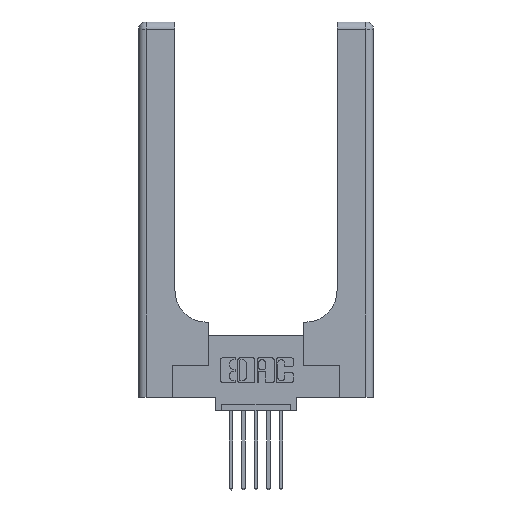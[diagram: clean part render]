
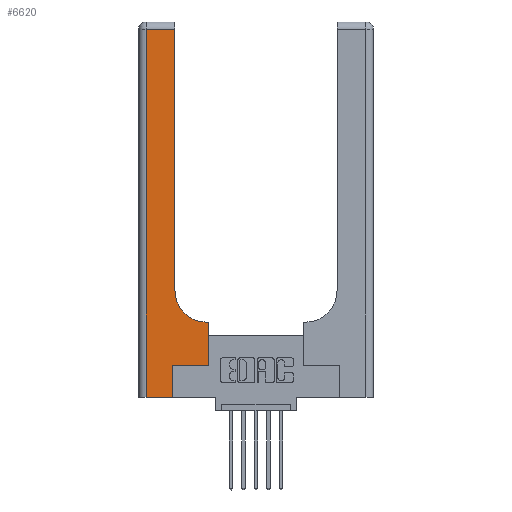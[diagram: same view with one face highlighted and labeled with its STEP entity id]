
A CAD part, top view. The second image highlights one B-rep face of the part: STEP entity #6620.
In plain terms, the highlighted planar face has unit normal (0, 0, 1).
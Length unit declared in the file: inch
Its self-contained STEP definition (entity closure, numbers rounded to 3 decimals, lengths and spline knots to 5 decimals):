
#94 = DIRECTION ( 'NONE',  ( 0., 1., 0. ) ) ;
#174 = EDGE_CURVE ( 'NONE', #13040, #5169, #3741, .T. ) ;
#616 = EDGE_CURVE ( 'NONE', #13150, #13040, #9345, .T. ) ;
#726 = EDGE_LOOP ( 'NONE', ( #3151, #6477, #8245, #13730, #7677, #1222, #13905, #7162, #2222 ) ) ;
#1222 = ORIENTED_EDGE ( 'NONE', *, *, #7306, .T. ) ;
#1320 = AXIS2_PLACEMENT_3D ( 'NONE', #1324, #11108, #4502 ) ;
#1324 = CARTESIAN_POINT ( 'NONE',  ( 0., 3., 0.37 ) ) ;
#1358 = CARTESIAN_POINT ( 'NONE',  ( 0.5585, 0.25, 0.37 ) ) ;
#1374 = VERTEX_POINT ( 'NONE', #5306 ) ;
#1387 = LINE ( 'NONE', #9585, #12266 ) ;
#1781 = VERTEX_POINT ( 'NONE', #8763 ) ;
#1799 = VECTOR ( 'NONE', #13992, 39.37008 ) ;
#1898 = CARTESIAN_POINT ( 'NONE',  ( 0.5415, 0.85, 0.37 ) ) ;
#2222 = ORIENTED_EDGE ( 'NONE', *, *, #8537, .T. ) ;
#2300 = PLANE ( 'NONE',  #1320 ) ;
#2305 = VECTOR ( 'NONE', #6820, 39.37008 ) ;
#2372 = DIRECTION ( 'NONE',  ( 0., 1., 0. ) ) ;
#2511 = CARTESIAN_POINT ( 'NONE',  ( 0.06, 3., 0.37 ) ) ;
#2556 = VECTOR ( 'NONE', #7871, 39.37008 ) ;
#2575 = LINE ( 'NONE', #1358, #9377 ) ;
#2824 = VERTEX_POINT ( 'NONE', #13608 ) ;
#2845 = DIRECTION ( 'NONE',  ( 0., 1., 0. ) ) ;
#3012 = CARTESIAN_POINT ( 'NONE',  ( 0.2915, 0.6, 0.37 ) ) ;
#3151 = ORIENTED_EDGE ( 'NONE', *, *, #4875, .T. ) ;
#3509 = CARTESIAN_POINT ( 'NONE',  ( 0.269, 0., 0.37 ) ) ;
#3741 = LINE ( 'NONE', #3509, #10190 ) ;
#4502 = DIRECTION ( 'NONE',  ( -1., 0., 0. ) ) ;
#4520 = EDGE_CURVE ( 'NONE', #1781, #4940, #12146, .T. ) ;
#4604 = EDGE_CURVE ( 'NONE', #2824, #13150, #5165, .T. ) ;
#4875 = EDGE_CURVE ( 'NONE', #10876, #1374, #8008, .T. ) ;
#4940 = VERTEX_POINT ( 'NONE', #5031 ) ;
#5031 = CARTESIAN_POINT ( 'NONE',  ( 0.5415, 0.6, 0.37 ) ) ;
#5098 = DIRECTION ( 'NONE',  ( 1., 0., 0. ) ) ;
#5165 = LINE ( 'NONE', #2511, #2305 ) ;
#5169 = VERTEX_POINT ( 'NONE', #8729 ) ;
#5306 = CARTESIAN_POINT ( 'NONE',  ( 0.2915, 2.94, 0.37 ) ) ;
#6075 = EDGE_CURVE ( 'NONE', #6850, #1781, #2575, .T. ) ;
#6453 = EDGE_CURVE ( 'NONE', #1374, #2824, #1387, .T. ) ;
#6477 = ORIENTED_EDGE ( 'NONE', *, *, #6453, .T. ) ;
#6620 = ADVANCED_FACE ( 'NONE', ( #9181 ), #2300, .F. ) ;
#6820 = DIRECTION ( 'NONE',  ( 0., -1., 0. ) ) ;
#6850 = VERTEX_POINT ( 'NONE', #10008 ) ;
#7162 = ORIENTED_EDGE ( 'NONE', *, *, #4520, .T. ) ;
#7306 = EDGE_CURVE ( 'NONE', #5169, #6850, #12441, .T. ) ;
#7318 = DIRECTION ( 'NONE',  ( -1., 0., 0. ) ) ;
#7677 = ORIENTED_EDGE ( 'NONE', *, *, #174, .T. ) ;
#7871 = DIRECTION ( 'NONE',  ( 1., 0., 0. ) ) ;
#8008 = LINE ( 'NONE', #12121, #12308 ) ;
#8105 = CARTESIAN_POINT ( 'NONE',  ( 0.269, 0., 0.37 ) ) ;
#8245 = ORIENTED_EDGE ( 'NONE', *, *, #4604, .T. ) ;
#8314 = CARTESIAN_POINT ( 'NONE',  ( 0.06, 0., 0.37 ) ) ;
#8537 = EDGE_CURVE ( 'NONE', #4940, #10876, #13397, .T. ) ;
#8729 = CARTESIAN_POINT ( 'NONE',  ( 0.269, 0.25, 0.37 ) ) ;
#8763 = CARTESIAN_POINT ( 'NONE',  ( 0.5585, 0.6, 0.37 ) ) ;
#8985 = CARTESIAN_POINT ( 'NONE',  ( 0., 0., 0.37 ) ) ;
#9181 = FACE_OUTER_BOUND ( 'NONE', #726, .T. ) ;
#9345 = LINE ( 'NONE', #8985, #2556 ) ;
#9377 = VECTOR ( 'NONE', #2372, 39.37008 ) ;
#9585 = CARTESIAN_POINT ( 'NONE',  ( 0., 2.94, 0.37 ) ) ;
#10008 = CARTESIAN_POINT ( 'NONE',  ( 0.5585, 0.25, 0.37 ) ) ;
#10190 = VECTOR ( 'NONE', #2845, 39.37008 ) ;
#10680 = CARTESIAN_POINT ( 'NONE',  ( 0.269, 0.25, 0.37 ) ) ;
#10876 = VERTEX_POINT ( 'NONE', #12803 ) ;
#11108 = DIRECTION ( 'NONE',  ( 0., 0., -1. ) ) ;
#11633 = DIRECTION ( 'NONE',  ( 0., 0., -1. ) ) ;
#11793 = DIRECTION ( 'NONE',  ( 1., 0., 0. ) ) ;
#12121 = CARTESIAN_POINT ( 'NONE',  ( 0.2915, 3., 0.37 ) ) ;
#12146 = LINE ( 'NONE', #3012, #1799 ) ;
#12266 = VECTOR ( 'NONE', #7318, 39.37008 ) ;
#12308 = VECTOR ( 'NONE', #94, 39.37008 ) ;
#12441 = LINE ( 'NONE', #10680, #13618 ) ;
#12803 = CARTESIAN_POINT ( 'NONE',  ( 0.2915, 0.85, 0.37 ) ) ;
#13040 = VERTEX_POINT ( 'NONE', #8105 ) ;
#13046 = AXIS2_PLACEMENT_3D ( 'NONE', #1898, #11633, #5098 ) ;
#13150 = VERTEX_POINT ( 'NONE', #8314 ) ;
#13397 = CIRCLE ( 'NONE', #13046, 0.25 ) ;
#13608 = CARTESIAN_POINT ( 'NONE',  ( 0.06, 2.94, 0.37 ) ) ;
#13618 = VECTOR ( 'NONE', #11793, 39.37008 ) ;
#13730 = ORIENTED_EDGE ( 'NONE', *, *, #616, .T. ) ;
#13905 = ORIENTED_EDGE ( 'NONE', *, *, #6075, .T. ) ;
#13992 = DIRECTION ( 'NONE',  ( -1., 0., 0. ) ) ;
